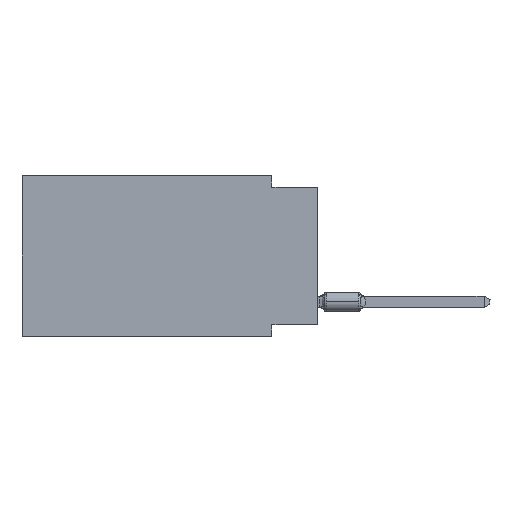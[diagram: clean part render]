
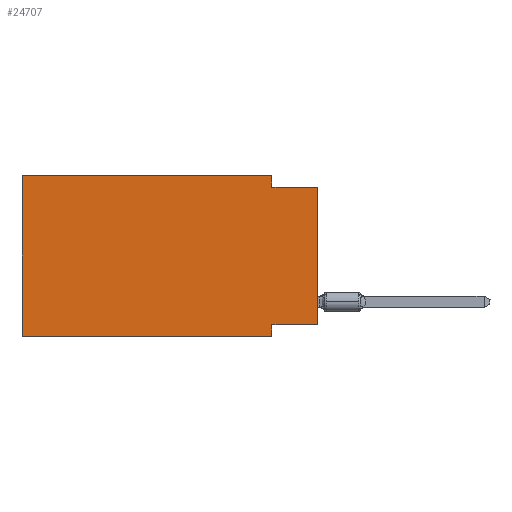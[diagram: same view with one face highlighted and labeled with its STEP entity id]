
A CAD part, left-side view. The second image highlights one B-rep face of the part: STEP entity #24707.
In plain terms, the highlighted planar face has unit normal (-1, 0, 0).
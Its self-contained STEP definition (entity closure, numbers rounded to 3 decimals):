
#833 = VECTOR ( 'NONE', #68775, 1000. ) ;
#998 = PLANE ( 'NONE',  #42851 ) ;
#1996 = EDGE_LOOP ( 'NONE', ( #79407, #57571, #59484, #75478, #79838, #7537, #50464, #61398 ) ) ;
#2846 = VECTOR ( 'NONE', #22938, 1000. ) ;
#4354 = VECTOR ( 'NONE', #11609, 1000. ) ;
#7537 = ORIENTED_EDGE ( 'NONE', *, *, #9158, .T. ) ;
#9158 = EDGE_CURVE ( 'NONE', #51057, #37143, #15398, .T. ) ;
#10443 = LINE ( 'NONE', #35556, #833 ) ;
#10574 = LINE ( 'NONE', #29514, #2846 ) ;
#10744 = CARTESIAN_POINT ( 'NONE',  ( 0., 0., -0.635 ) ) ;
#11298 = VECTOR ( 'NONE', #26113, 1000. ) ;
#11609 = DIRECTION ( 'NONE',  ( 0., -1., 0. ) ) ;
#12519 = LINE ( 'NONE', #31071, #11298 ) ;
#14133 = CARTESIAN_POINT ( 'NONE',  ( 0., 2.54, -0.635 ) ) ;
#14622 = CARTESIAN_POINT ( 'NONE',  ( 0., 0., -0.635 ) ) ;
#14793 = VECTOR ( 'NONE', #79199, 1000. ) ;
#15272 = DIRECTION ( 'NONE',  ( 0., 0., -1. ) ) ;
#15398 = LINE ( 'NONE', #35141, #14793 ) ;
#16942 = LINE ( 'NONE', #10744, #38081 ) ;
#17791 = LINE ( 'NONE', #68044, #4354 ) ;
#18688 = DIRECTION ( 'NONE',  ( 1., 0., 0. ) ) ;
#19680 = CARTESIAN_POINT ( 'NONE',  ( 0., 16.383, -8.89 ) ) ;
#21918 = CARTESIAN_POINT ( 'NONE',  ( 0., 2.54, 0. ) ) ;
#22938 = DIRECTION ( 'NONE',  ( 0., 0., 1. ) ) ;
#24707 = ADVANCED_FACE ( 'NONE', ( #25280 ), #998, .F. ) ;
#24723 = EDGE_CURVE ( 'NONE', #35726, #37143, #12519, .T. ) ;
#25280 = FACE_OUTER_BOUND ( 'NONE', #1996, .T. ) ;
#26113 = DIRECTION ( 'NONE',  ( 0., 0., -1. ) ) ;
#26286 = CARTESIAN_POINT ( 'NONE',  ( 0., 0., -8.255 ) ) ;
#28838 = LINE ( 'NONE', #53963, #33091 ) ;
#29514 = CARTESIAN_POINT ( 'NONE',  ( 0., 0., 0. ) ) ;
#31071 = CARTESIAN_POINT ( 'NONE',  ( 0., 2.54, -8.89 ) ) ;
#33091 = VECTOR ( 'NONE', #15272, 1000. ) ;
#35091 = EDGE_CURVE ( 'NONE', #39426, #38149, #10574, .T. ) ;
#35141 = CARTESIAN_POINT ( 'NONE',  ( 0., 16.383, -8.89 ) ) ;
#35556 = CARTESIAN_POINT ( 'NONE',  ( 0., 0., -8.255 ) ) ;
#35726 = VERTEX_POINT ( 'NONE', #53574 ) ;
#37087 = EDGE_CURVE ( 'NONE', #66580, #49443, #17791, .T. ) ;
#37143 = VERTEX_POINT ( 'NONE', #44947 ) ;
#38081 = VECTOR ( 'NONE', #74591, 1000. ) ;
#38149 = VERTEX_POINT ( 'NONE', #14622 ) ;
#39426 = VERTEX_POINT ( 'NONE', #26286 ) ;
#41950 = EDGE_CURVE ( 'NONE', #39426, #35726, #10443, .T. ) ;
#42851 = AXIS2_PLACEMENT_3D ( 'NONE', #81338, #18688, #43814 ) ;
#43353 = VERTEX_POINT ( 'NONE', #14133 ) ;
#43814 = DIRECTION ( 'NONE',  ( 0., 0., -1. ) ) ;
#44947 = CARTESIAN_POINT ( 'NONE',  ( 0., 2.54, -8.89 ) ) ;
#46765 = LINE ( 'NONE', #52935, #76689 ) ;
#49443 = VERTEX_POINT ( 'NONE', #21918 ) ;
#50464 = ORIENTED_EDGE ( 'NONE', *, *, #24723, .F. ) ;
#51057 = VERTEX_POINT ( 'NONE', #19680 ) ;
#51507 = CARTESIAN_POINT ( 'NONE',  ( 0., 16.383, 0. ) ) ;
#52935 = CARTESIAN_POINT ( 'NONE',  ( 0., 16.383, 0. ) ) ;
#53574 = CARTESIAN_POINT ( 'NONE',  ( 0., 2.54, -8.255 ) ) ;
#53963 = CARTESIAN_POINT ( 'NONE',  ( 0., 2.54, 0. ) ) ;
#57571 = ORIENTED_EDGE ( 'NONE', *, *, #62153, .F. ) ;
#59484 = ORIENTED_EDGE ( 'NONE', *, *, #78522, .F. ) ;
#61398 = ORIENTED_EDGE ( 'NONE', *, *, #41950, .F. ) ;
#62153 = EDGE_CURVE ( 'NONE', #43353, #38149, #16942, .T. ) ;
#64566 = EDGE_CURVE ( 'NONE', #51057, #66580, #46765, .T. ) ;
#66580 = VERTEX_POINT ( 'NONE', #51507 ) ;
#68044 = CARTESIAN_POINT ( 'NONE',  ( 0., 16.383, 0. ) ) ;
#68775 = DIRECTION ( 'NONE',  ( 0., 1., 0. ) ) ;
#71904 = DIRECTION ( 'NONE',  ( 0., 0., 1. ) ) ;
#74591 = DIRECTION ( 'NONE',  ( 0., -1., 0. ) ) ;
#75478 = ORIENTED_EDGE ( 'NONE', *, *, #37087, .F. ) ;
#76689 = VECTOR ( 'NONE', #71904, 1000. ) ;
#78522 = EDGE_CURVE ( 'NONE', #49443, #43353, #28838, .T. ) ;
#79199 = DIRECTION ( 'NONE',  ( 0., -1., 0. ) ) ;
#79407 = ORIENTED_EDGE ( 'NONE', *, *, #35091, .T. ) ;
#79838 = ORIENTED_EDGE ( 'NONE', *, *, #64566, .F. ) ;
#81338 = CARTESIAN_POINT ( 'NONE',  ( 0., 16.383, 0. ) ) ;
